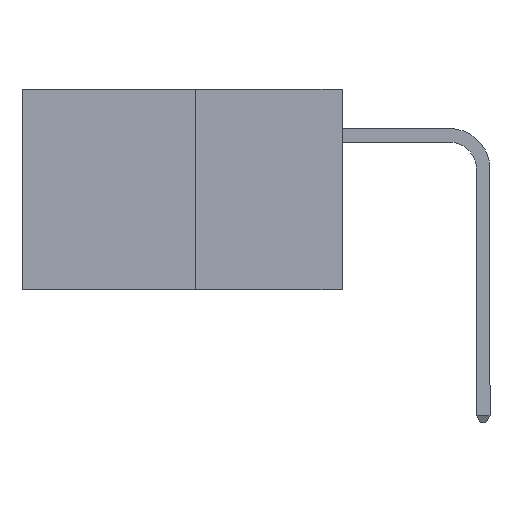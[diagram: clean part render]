
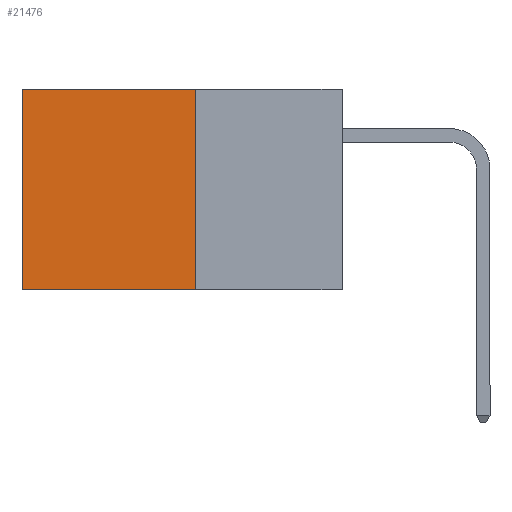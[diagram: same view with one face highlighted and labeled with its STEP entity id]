
A CAD part, left-side view. The second image highlights one B-rep face of the part: STEP entity #21476.
In plain terms, the highlighted planar face has unit normal (-1, 0, 0).
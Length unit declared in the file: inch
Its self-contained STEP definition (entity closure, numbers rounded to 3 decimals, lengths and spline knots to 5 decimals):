
#644 = CARTESIAN_POINT ( 'NONE',  ( 0.277, 0.27, -0.37 ) ) ;
#1465 = DIRECTION ( 'NONE',  ( 0., 0., -1. ) ) ;
#2313 = DIRECTION ( 'NONE',  ( 0., 1., 0. ) ) ;
#2627 = DIRECTION ( 'NONE',  ( 1., 0., 0. ) ) ;
#2741 = CARTESIAN_POINT ( 'NONE',  ( 0.277, 0.27, 0. ) ) ;
#3206 = VERTEX_POINT ( 'NONE', #2741 ) ;
#4553 = FACE_OUTER_BOUND ( 'NONE', #19110, .T. ) ;
#4592 = DIRECTION ( 'NONE',  ( 0., 1., 0. ) ) ;
#4932 = VERTEX_POINT ( 'NONE', #21564 ) ;
#6619 = CARTESIAN_POINT ( 'NONE',  ( 0.277, 0.59, -0.37 ) ) ;
#7888 = VERTEX_POINT ( 'NONE', #10588 ) ;
#8303 = ORIENTED_EDGE ( 'NONE', *, *, #8426, .T. ) ;
#8426 = EDGE_CURVE ( 'NONE', #7888, #9124, #25038, .T. ) ;
#9124 = VERTEX_POINT ( 'NONE', #6619 ) ;
#10394 = AXIS2_PLACEMENT_3D ( 'NONE', #644, #2627, #16556 ) ;
#10588 = CARTESIAN_POINT ( 'NONE',  ( 0.277, 0.59, 0. ) ) ;
#12015 = CARTESIAN_POINT ( 'NONE',  ( 0.277, 0.59, -0.37 ) ) ;
#12016 = EDGE_CURVE ( 'NONE', #3206, #7888, #14475, .T. ) ;
#12222 = CARTESIAN_POINT ( 'NONE',  ( 0.277, 0.27, 0. ) ) ;
#12527 = PLANE ( 'NONE',  #10394 ) ;
#13335 = CARTESIAN_POINT ( 'NONE',  ( 0.277, 0.27, -0.37 ) ) ;
#13692 = ORIENTED_EDGE ( 'NONE', *, *, #12016, .T. ) ;
#13834 = VECTOR ( 'NONE', #2313, 39.37008 ) ;
#14475 = LINE ( 'NONE', #12222, #13834 ) ;
#14876 = ORIENTED_EDGE ( 'NONE', *, *, #18833, .F. ) ;
#16020 = DIRECTION ( 'NONE',  ( 0., 0., -1. ) ) ;
#16556 = DIRECTION ( 'NONE',  ( 0., 0., -1. ) ) ;
#17031 = EDGE_CURVE ( 'NONE', #4932, #9124, #20051, .T. ) ;
#17455 = VECTOR ( 'NONE', #1465, 39.37008 ) ;
#18773 = ORIENTED_EDGE ( 'NONE', *, *, #17031, .F. ) ;
#18833 = EDGE_CURVE ( 'NONE', #3206, #4932, #22754, .T. ) ;
#19110 = EDGE_LOOP ( 'NONE', ( #8303, #18773, #14876, #13692 ) ) ;
#19735 = VECTOR ( 'NONE', #16020, 39.37008 ) ;
#20051 = LINE ( 'NONE', #20493, #24095 ) ;
#20493 = CARTESIAN_POINT ( 'NONE',  ( 0.277, 0.27, -0.37 ) ) ;
#21476 = ADVANCED_FACE ( 'NONE', ( #4553 ), #12527, .F. ) ;
#21564 = CARTESIAN_POINT ( 'NONE',  ( 0.277, 0.27, -0.37 ) ) ;
#22754 = LINE ( 'NONE', #13335, #17455 ) ;
#24095 = VECTOR ( 'NONE', #4592, 39.37008 ) ;
#25038 = LINE ( 'NONE', #12015, #19735 ) ;
